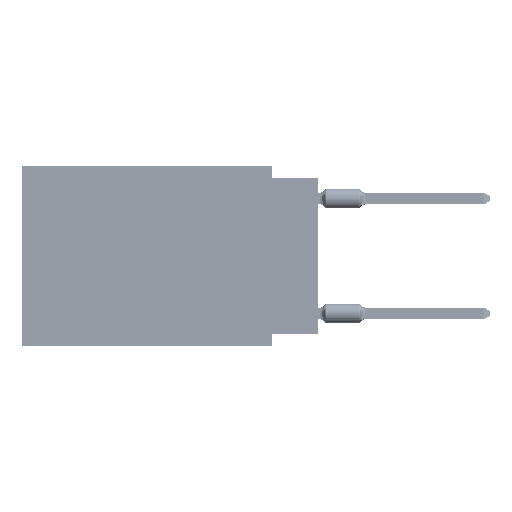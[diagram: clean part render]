
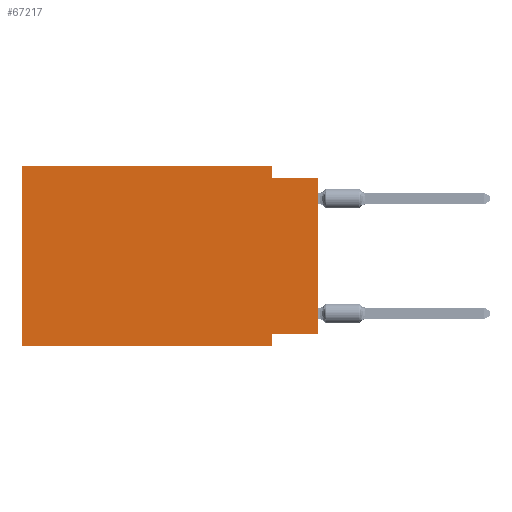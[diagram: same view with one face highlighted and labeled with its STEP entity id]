
A CAD part, left-side view. The second image highlights one B-rep face of the part: STEP entity #67217.
In plain terms, the highlighted planar face has unit normal (-1, 0, 0).
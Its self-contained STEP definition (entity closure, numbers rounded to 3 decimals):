
#3177 = PLANE ( 'NONE',  #6362 ) ;
#3946 = ORIENTED_EDGE ( 'NONE', *, *, #56280, .F. ) ;
#4233 = EDGE_CURVE ( 'NONE', #80641, #59659, #48654, .T. ) ;
#6197 = ORIENTED_EDGE ( 'NONE', *, *, #65415, .F. ) ;
#6362 = AXIS2_PLACEMENT_3D ( 'NONE', #35947, #9502, #29689 ) ;
#9108 = CARTESIAN_POINT ( 'NONE',  ( 0., 2.54, 0. ) ) ;
#9259 = VECTOR ( 'NONE', #54499, 1000. ) ;
#9363 = ORIENTED_EDGE ( 'NONE', *, *, #67271, .T. ) ;
#9502 = DIRECTION ( 'NONE',  ( 1., 0., 0. ) ) ;
#10125 = EDGE_CURVE ( 'NONE', #65434, #56947, #74362, .T. ) ;
#11936 = DIRECTION ( 'NONE',  ( 0., 1., 0. ) ) ;
#14633 = VERTEX_POINT ( 'NONE', #47150 ) ;
#14859 = LINE ( 'NONE', #62806, #32256 ) ;
#15346 = DIRECTION ( 'NONE',  ( 0., -1., 0. ) ) ;
#18639 = LINE ( 'NONE', #73340, #67691 ) ;
#21994 = ORIENTED_EDGE ( 'NONE', *, *, #74469, .F. ) ;
#24049 = CARTESIAN_POINT ( 'NONE',  ( 0., 2.54, -9.271 ) ) ;
#25700 = VECTOR ( 'NONE', #68087, 1000. ) ;
#26127 = EDGE_CURVE ( 'NONE', #14633, #80641, #18639, .T. ) ;
#29314 = VECTOR ( 'NONE', #15346, 1000. ) ;
#29649 = CARTESIAN_POINT ( 'NONE',  ( 0., 0., -0.635 ) ) ;
#29689 = DIRECTION ( 'NONE',  ( 0., 0., -1. ) ) ;
#32256 = VECTOR ( 'NONE', #61032, 1000. ) ;
#35947 = CARTESIAN_POINT ( 'NONE',  ( 0., 16.383, 0. ) ) ;
#37340 = LINE ( 'NONE', #9108, #37641 ) ;
#37641 = VECTOR ( 'NONE', #43623, 1000. ) ;
#38417 = VECTOR ( 'NONE', #66112, 1000. ) ;
#40072 = LINE ( 'NONE', #67409, #38417 ) ;
#40596 = CARTESIAN_POINT ( 'NONE',  ( 0., 16.383, 0. ) ) ;
#42487 = ORIENTED_EDGE ( 'NONE', *, *, #26127, .F. ) ;
#43623 = DIRECTION ( 'NONE',  ( 0., 0., -1. ) ) ;
#43894 = EDGE_CURVE ( 'NONE', #14633, #56947, #14859, .T. ) ;
#44273 = VERTEX_POINT ( 'NONE', #45074 ) ;
#45074 = CARTESIAN_POINT ( 'NONE',  ( 0., 16.383, 0. ) ) ;
#46686 = CARTESIAN_POINT ( 'NONE',  ( 0., 2.54, -0.635 ) ) ;
#47150 = CARTESIAN_POINT ( 'NONE',  ( 0., 0., -9.271 ) ) ;
#48211 = DIRECTION ( 'NONE',  ( 0., -1., 0. ) ) ;
#48654 = LINE ( 'NONE', #83167, #9259 ) ;
#50541 = VECTOR ( 'NONE', #48211, 1000. ) ;
#53586 = ORIENTED_EDGE ( 'NONE', *, *, #10125, .F. ) ;
#54467 = VERTEX_POINT ( 'NONE', #65762 ) ;
#54499 = DIRECTION ( 'NONE',  ( 0., 0., -1. ) ) ;
#54519 = ORIENTED_EDGE ( 'NONE', *, *, #4233, .F. ) ;
#56280 = EDGE_CURVE ( 'NONE', #81712, #44273, #40072, .T. ) ;
#56947 = VERTEX_POINT ( 'NONE', #29649 ) ;
#59556 = ORIENTED_EDGE ( 'NONE', *, *, #43894, .T. ) ;
#59659 = VERTEX_POINT ( 'NONE', #81385 ) ;
#61032 = DIRECTION ( 'NONE',  ( 0., 0., 1. ) ) ;
#62806 = CARTESIAN_POINT ( 'NONE',  ( 0., 0., 0. ) ) ;
#65415 = EDGE_CURVE ( 'NONE', #54467, #65434, #37340, .T. ) ;
#65434 = VERTEX_POINT ( 'NONE', #46686 ) ;
#65762 = CARTESIAN_POINT ( 'NONE',  ( 0., 2.54, 0. ) ) ;
#66112 = DIRECTION ( 'NONE',  ( 0., 0., 1. ) ) ;
#67217 = ADVANCED_FACE ( 'NONE', ( #85246 ), #3177, .F. ) ;
#67271 = EDGE_CURVE ( 'NONE', #81712, #59659, #76747, .T. ) ;
#67409 = CARTESIAN_POINT ( 'NONE',  ( 0., 16.383, 0. ) ) ;
#67500 = LINE ( 'NONE', #40596, #50541 ) ;
#67691 = VECTOR ( 'NONE', #11936, 1000. ) ;
#68087 = DIRECTION ( 'NONE',  ( 0., -1., 0. ) ) ;
#69194 = EDGE_LOOP ( 'NONE', ( #59556, #53586, #6197, #21994, #3946, #9363, #54519, #42487 ) ) ;
#73053 = CARTESIAN_POINT ( 'NONE',  ( 0., 0., -0.635 ) ) ;
#73340 = CARTESIAN_POINT ( 'NONE',  ( 0., 0., -9.271 ) ) ;
#74362 = LINE ( 'NONE', #73053, #25700 ) ;
#74469 = EDGE_CURVE ( 'NONE', #44273, #54467, #67500, .T. ) ;
#76747 = LINE ( 'NONE', #77186, #29314 ) ;
#77186 = CARTESIAN_POINT ( 'NONE',  ( 0., 16.383, -9.906 ) ) ;
#80641 = VERTEX_POINT ( 'NONE', #24049 ) ;
#81385 = CARTESIAN_POINT ( 'NONE',  ( 0., 2.54, -9.906 ) ) ;
#81712 = VERTEX_POINT ( 'NONE', #88422 ) ;
#83167 = CARTESIAN_POINT ( 'NONE',  ( 0., 2.54, -9.906 ) ) ;
#85246 = FACE_OUTER_BOUND ( 'NONE', #69194, .T. ) ;
#88422 = CARTESIAN_POINT ( 'NONE',  ( 0., 16.383, -9.906 ) ) ;
